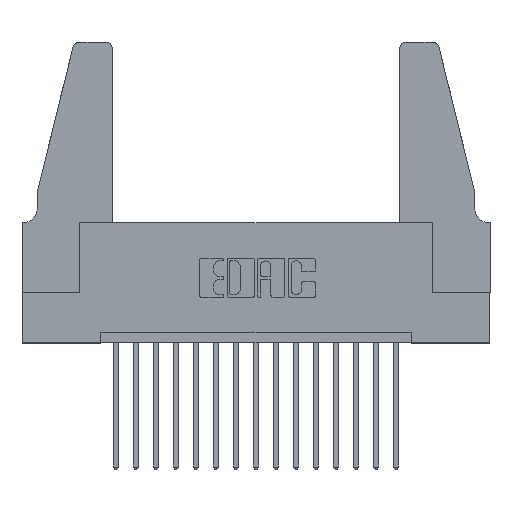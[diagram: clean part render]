
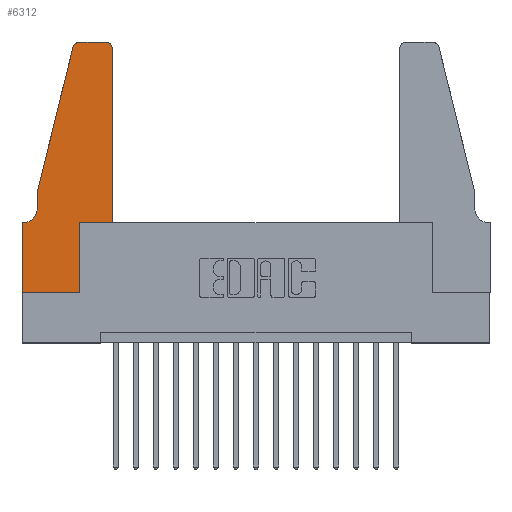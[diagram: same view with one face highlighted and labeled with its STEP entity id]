
A CAD part, top view. The second image highlights one B-rep face of the part: STEP entity #6312.
In plain terms, the highlighted planar face has unit normal (0, 0, 1).
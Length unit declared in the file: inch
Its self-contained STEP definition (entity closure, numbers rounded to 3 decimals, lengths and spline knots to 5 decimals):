
#330 = ORIENTED_EDGE ( 'NONE', *, *, #9269, .T. ) ;
#601 = CARTESIAN_POINT ( 'NONE',  ( 0.284, 1.22, 0.37 ) ) ;
#619 = EDGE_CURVE ( 'NONE', #6105, #16322, #8445, .T. ) ;
#624 = EDGE_LOOP ( 'NONE', ( #11618, #11407, #14547, #7009, #2710, #1346, #15586, #330, #12214, #13468, #14137, #8501 ) ) ;
#644 = PLANE ( 'NONE',  #5753 ) ;
#945 = VERTEX_POINT ( 'NONE', #9241 ) ;
#987 = LINE ( 'NONE', #13956, #7127 ) ;
#1346 = ORIENTED_EDGE ( 'NONE', *, *, #619, .T. ) ;
#1653 = CARTESIAN_POINT ( 'NONE',  ( 0.4205, 1.22, 0.37 ) ) ;
#1829 = EDGE_CURVE ( 'NONE', #15953, #13426, #7566, .T. ) ;
#1990 = DIRECTION ( 'NONE',  ( 1., 0., 0. ) ) ;
#2090 = DIRECTION ( 'NONE',  ( -1., 0., 0. ) ) ;
#2129 = EDGE_CURVE ( 'NONE', #16322, #10834, #13122, .T. ) ;
#2271 = CARTESIAN_POINT ( 'NONE',  ( 0.25487, 1.22718, 0.37 ) ) ;
#2327 = LINE ( 'NONE', #14112, #9333 ) ;
#2346 = CARTESIAN_POINT ( 'NONE',  ( 0.2865, 0., 0.37 ) ) ;
#2354 = EDGE_CURVE ( 'NONE', #2999, #5936, #5887, .T. ) ;
#2516 = EDGE_CURVE ( 'NONE', #5936, #13274, #7548, .T. ) ;
#2710 = ORIENTED_EDGE ( 'NONE', *, *, #9197, .T. ) ;
#2999 = VERTEX_POINT ( 'NONE', #11791 ) ;
#3064 = CARTESIAN_POINT ( 'NONE',  ( 0.0055, 0.35, 0.37 ) ) ;
#3349 = FACE_OUTER_BOUND ( 'NONE', #624, .T. ) ;
#3643 = CARTESIAN_POINT ( 'NONE',  ( 0.284, 1.25, 0.37 ) ) ;
#4229 = DIRECTION ( 'NONE',  ( 1., 0., 0. ) ) ;
#4253 = VECTOR ( 'NONE', #13341, 39.37008 ) ;
#4391 = DIRECTION ( 'NONE',  ( 0., 0., 1. ) ) ;
#4614 = DIRECTION ( 'NONE',  ( 1., 0., 0. ) ) ;
#4641 = CARTESIAN_POINT ( 'NONE',  ( 0.0755, 0.5, 0.37 ) ) ;
#5742 = LINE ( 'NONE', #6792, #8657 ) ;
#5753 = AXIS2_PLACEMENT_3D ( 'NONE', #16340, #9855, #1990 ) ;
#5756 = CARTESIAN_POINT ( 'NONE',  ( 0.0755, 0.35, 0.37 ) ) ;
#5887 = LINE ( 'NONE', #10425, #16879 ) ;
#5889 = VERTEX_POINT ( 'NONE', #2346 ) ;
#5936 = VERTEX_POINT ( 'NONE', #13257 ) ;
#6105 = VERTEX_POINT ( 'NONE', #3064 ) ;
#6170 = DIRECTION ( 'NONE',  ( -1., 0., 0. ) ) ;
#6228 = DIRECTION ( 'NONE',  ( -0.239, -0.971, 0. ) ) ;
#6312 = ADVANCED_FACE ( 'NONE', ( #3349 ), #644, .T. ) ;
#6679 = VERTEX_POINT ( 'NONE', #3643 ) ;
#6792 = CARTESIAN_POINT ( 'NONE',  ( 0.2865, 0.35, 0.37 ) ) ;
#6946 = VECTOR ( 'NONE', #6228, 39.37008 ) ;
#7009 = ORIENTED_EDGE ( 'NONE', *, *, #10259, .T. ) ;
#7127 = VECTOR ( 'NONE', #2090, 39.37008 ) ;
#7130 = CARTESIAN_POINT ( 'NONE',  ( 0., 0., 0.37 ) ) ;
#7534 = VERTEX_POINT ( 'NONE', #15557 ) ;
#7548 = LINE ( 'NONE', #11976, #4253 ) ;
#7566 = LINE ( 'NONE', #7787, #6946 ) ;
#7787 = CARTESIAN_POINT ( 'NONE',  ( 0.0755, 0.5, 0.37 ) ) ;
#8208 = DIRECTION ( 'NONE',  ( 0., 0., 1. ) ) ;
#8445 = LINE ( 'NONE', #5756, #11759 ) ;
#8501 = ORIENTED_EDGE ( 'NONE', *, *, #12593, .T. ) ;
#8546 = EDGE_CURVE ( 'NONE', #6679, #15953, #14000, .T. ) ;
#8657 = VECTOR ( 'NONE', #11887, 39.37008 ) ;
#9197 = EDGE_CURVE ( 'NONE', #7534, #6105, #10865, .T. ) ;
#9241 = CARTESIAN_POINT ( 'NONE',  ( 0.4205, 1.25, 0.37 ) ) ;
#9269 = EDGE_CURVE ( 'NONE', #10834, #5889, #16058, .T. ) ;
#9333 = VECTOR ( 'NONE', #15454, 39.37008 ) ;
#9634 = EDGE_CURVE ( 'NONE', #945, #6679, #987, .T. ) ;
#9855 = DIRECTION ( 'NONE',  ( 0., 0., 1. ) ) ;
#9935 = DIRECTION ( 'NONE',  ( 0., 0., -1. ) ) ;
#10259 = EDGE_CURVE ( 'NONE', #13426, #7534, #2327, .T. ) ;
#10425 = CARTESIAN_POINT ( 'NONE',  ( 0.4505, 0.35, 0.37 ) ) ;
#10827 = CARTESIAN_POINT ( 'NONE',  ( 0.4505, 1.22, 0.37 ) ) ;
#10834 = VERTEX_POINT ( 'NONE', #16224 ) ;
#10865 = CIRCLE ( 'NONE', #13087, 0.07 ) ;
#11319 = EDGE_CURVE ( 'NONE', #5889, #2999, #5742, .T. ) ;
#11407 = ORIENTED_EDGE ( 'NONE', *, *, #8546, .T. ) ;
#11618 = ORIENTED_EDGE ( 'NONE', *, *, #9634, .T. ) ;
#11759 = VECTOR ( 'NONE', #6170, 39.37008 ) ;
#11791 = CARTESIAN_POINT ( 'NONE',  ( 0.2865, 0.35, 0.37 ) ) ;
#11887 = DIRECTION ( 'NONE',  ( 0., 1., 0. ) ) ;
#11976 = CARTESIAN_POINT ( 'NONE',  ( 0.4505, 0.35, 0.37 ) ) ;
#12214 = ORIENTED_EDGE ( 'NONE', *, *, #11319, .T. ) ;
#12504 = VECTOR ( 'NONE', #4614, 39.37008 ) ;
#12593 = EDGE_CURVE ( 'NONE', #13274, #945, #15656, .T. ) ;
#13087 = AXIS2_PLACEMENT_3D ( 'NONE', #16332, #9935, #16484 ) ;
#13122 = LINE ( 'NONE', #7130, #16462 ) ;
#13181 = AXIS2_PLACEMENT_3D ( 'NONE', #1653, #8208, #4229 ) ;
#13257 = CARTESIAN_POINT ( 'NONE',  ( 0.4505, 0.35, 0.37 ) ) ;
#13274 = VERTEX_POINT ( 'NONE', #10827 ) ;
#13341 = DIRECTION ( 'NONE',  ( 0., 1., 0. ) ) ;
#13426 = VERTEX_POINT ( 'NONE', #4641 ) ;
#13468 = ORIENTED_EDGE ( 'NONE', *, *, #2354, .T. ) ;
#13956 = CARTESIAN_POINT ( 'NONE',  ( 0.2605, 1.25, 0.37 ) ) ;
#14000 = CIRCLE ( 'NONE', #15879, 0.03 ) ;
#14093 = CARTESIAN_POINT ( 'NONE',  ( 0., 0., 0.37 ) ) ;
#14112 = CARTESIAN_POINT ( 'NONE',  ( 0.0755, 0.5, 0.37 ) ) ;
#14137 = ORIENTED_EDGE ( 'NONE', *, *, #2516, .T. ) ;
#14547 = ORIENTED_EDGE ( 'NONE', *, *, #1829, .T. ) ;
#15112 = DIRECTION ( 'NONE',  ( 0., -1., 0. ) ) ;
#15454 = DIRECTION ( 'NONE',  ( 0., -1., 0. ) ) ;
#15557 = CARTESIAN_POINT ( 'NONE',  ( 0.0755, 0.42, 0.37 ) ) ;
#15586 = ORIENTED_EDGE ( 'NONE', *, *, #2129, .T. ) ;
#15656 = CIRCLE ( 'NONE', #13181, 0.03 ) ;
#15879 = AXIS2_PLACEMENT_3D ( 'NONE', #601, #4391, #16468 ) ;
#15928 = CARTESIAN_POINT ( 'NONE',  ( 0., 0.35, 0.37 ) ) ;
#15953 = VERTEX_POINT ( 'NONE', #2271 ) ;
#16058 = LINE ( 'NONE', #14093, #12504 ) ;
#16224 = CARTESIAN_POINT ( 'NONE',  ( 0., 0., 0.37 ) ) ;
#16322 = VERTEX_POINT ( 'NONE', #15928 ) ;
#16332 = CARTESIAN_POINT ( 'NONE',  ( 0.0055, 0.42, 0.37 ) ) ;
#16340 = CARTESIAN_POINT ( 'NONE',  ( 0., 0.35, 0.37 ) ) ;
#16462 = VECTOR ( 'NONE', #15112, 39.37008 ) ;
#16468 = DIRECTION ( 'NONE',  ( 1., 0., 0. ) ) ;
#16484 = DIRECTION ( 'NONE',  ( -1., 0., 0. ) ) ;
#16865 = DIRECTION ( 'NONE',  ( 1., 0., 0. ) ) ;
#16879 = VECTOR ( 'NONE', #16865, 39.37008 ) ;
